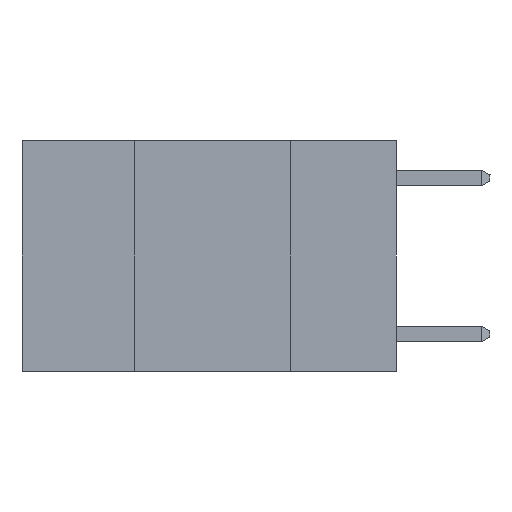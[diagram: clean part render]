
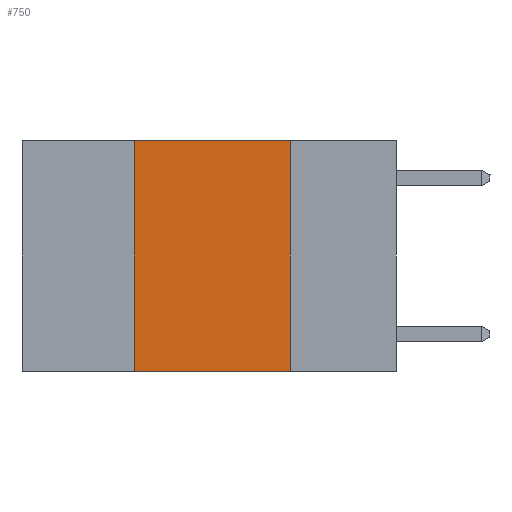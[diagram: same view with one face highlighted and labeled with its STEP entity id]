
A CAD part, left-side view. The second image highlights one B-rep face of the part: STEP entity #750.
In plain terms, the highlighted planar face has unit normal (-1, 0, 0).
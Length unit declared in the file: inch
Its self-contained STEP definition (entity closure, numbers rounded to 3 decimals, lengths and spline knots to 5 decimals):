
#438 = VERTEX_POINT ( 'NONE', #1815 ) ;
#750 = ADVANCED_FACE ( 'NONE', ( #5416 ), #2154, .F. ) ;
#1081 = CARTESIAN_POINT ( 'NONE',  ( 0., 0.17, 0. ) ) ;
#1311 = VERTEX_POINT ( 'NONE', #3632 ) ;
#1354 = CARTESIAN_POINT ( 'NONE',  ( 0., 0.42, 0. ) ) ;
#1518 = EDGE_CURVE ( 'NONE', #3741, #2138, #4677, .T. ) ;
#1524 = LINE ( 'NONE', #1354, #7920 ) ;
#1773 = EDGE_LOOP ( 'NONE', ( #4114, #2436, #7982, #6604 ) ) ;
#1815 = CARTESIAN_POINT ( 'NONE',  ( 0., 0.17, 0. ) ) ;
#1871 = CARTESIAN_POINT ( 'NONE',  ( 0., 0.42, -0.37 ) ) ;
#2077 = DIRECTION ( 'NONE',  ( 0., -1., 0. ) ) ;
#2138 = VERTEX_POINT ( 'NONE', #4115 ) ;
#2154 = PLANE ( 'NONE',  #8244 ) ;
#2268 = LINE ( 'NONE', #7460, #5557 ) ;
#2436 = ORIENTED_EDGE ( 'NONE', *, *, #4931, .F. ) ;
#3632 = CARTESIAN_POINT ( 'NONE',  ( 0., 0.42, 0. ) ) ;
#3741 = VERTEX_POINT ( 'NONE', #1871 ) ;
#3971 = DIRECTION ( 'NONE',  ( 0., 0., 1. ) ) ;
#4114 = ORIENTED_EDGE ( 'NONE', *, *, #4998, .F. ) ;
#4115 = CARTESIAN_POINT ( 'NONE',  ( 0., 0.17, -0.37 ) ) ;
#4392 = DIRECTION ( 'NONE',  ( 0., -1., 0. ) ) ;
#4677 = LINE ( 'NONE', #7950, #6929 ) ;
#4931 = EDGE_CURVE ( 'NONE', #1311, #438, #2268, .T. ) ;
#4998 = EDGE_CURVE ( 'NONE', #438, #2138, #6906, .T. ) ;
#5416 = FACE_OUTER_BOUND ( 'NONE', #1773, .T. ) ;
#5557 = VECTOR ( 'NONE', #4392, 39.37008 ) ;
#5668 = DIRECTION ( 'NONE',  ( 1., 0., 0. ) ) ;
#6269 = DIRECTION ( 'NONE',  ( 0., 0., -1. ) ) ;
#6604 = ORIENTED_EDGE ( 'NONE', *, *, #1518, .T. ) ;
#6660 = CARTESIAN_POINT ( 'NONE',  ( 0., 0.6, 0. ) ) ;
#6732 = EDGE_CURVE ( 'NONE', #3741, #1311, #1524, .T. ) ;
#6906 = LINE ( 'NONE', #1081, #7619 ) ;
#6929 = VECTOR ( 'NONE', #2077, 39.37008 ) ;
#7460 = CARTESIAN_POINT ( 'NONE',  ( 0., 0.6, 0. ) ) ;
#7619 = VECTOR ( 'NONE', #6269, 39.37008 ) ;
#7920 = VECTOR ( 'NONE', #3971, 39.37008 ) ;
#7950 = CARTESIAN_POINT ( 'NONE',  ( 0., 0.6, -0.37 ) ) ;
#7982 = ORIENTED_EDGE ( 'NONE', *, *, #6732, .F. ) ;
#8112 = DIRECTION ( 'NONE',  ( 0., 0., -1. ) ) ;
#8244 = AXIS2_PLACEMENT_3D ( 'NONE', #6660, #5668, #8112 ) ;
